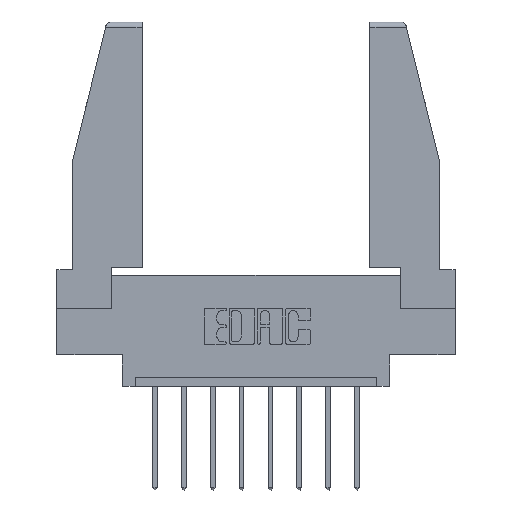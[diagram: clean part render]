
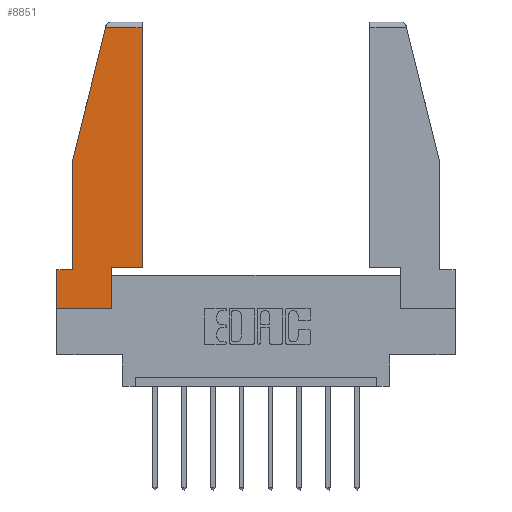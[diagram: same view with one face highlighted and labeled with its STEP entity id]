
A CAD part, top view. The second image highlights one B-rep face of the part: STEP entity #8851.
In plain terms, the highlighted planar face has unit normal (0, 0, 1).
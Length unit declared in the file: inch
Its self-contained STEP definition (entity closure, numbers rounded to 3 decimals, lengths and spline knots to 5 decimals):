
#19 = ORIENTED_EDGE ( 'NONE', *, *, #1486, .T. ) ;
#105 = CARTESIAN_POINT ( 'NONE',  ( 0.297, 0.223, 0. ) ) ;
#138 = LINE ( 'NONE', #12350, #1554 ) ;
#540 = ORIENTED_EDGE ( 'NONE', *, *, #1920, .T. ) ;
#546 = DIRECTION ( 'NONE',  ( 1., 0., 0. ) ) ;
#933 = LINE ( 'NONE', #105, #10803 ) ;
#965 = VERTEX_POINT ( 'NONE', #9725 ) ;
#1338 = CARTESIAN_POINT ( 'NONE',  ( 0.461, 0.223, 0. ) ) ;
#1431 = DIRECTION ( 'NONE',  ( 1., 0., 0. ) ) ;
#1440 = CARTESIAN_POINT ( 'NONE',  ( 0., 0.21, 0. ) ) ;
#1448 = ORIENTED_EDGE ( 'NONE', *, *, #9205, .T. ) ;
#1486 = EDGE_CURVE ( 'NONE', #11310, #4873, #933, .T. ) ;
#1554 = VECTOR ( 'NONE', #1431, 39.37008 ) ;
#1853 = VERTEX_POINT ( 'NONE', #2772 ) ;
#1867 = VERTEX_POINT ( 'NONE', #6920 ) ;
#1920 = EDGE_CURVE ( 'NONE', #4439, #10776, #9570, .T. ) ;
#1997 = DIRECTION ( 'NONE',  ( 0., -1., 0. ) ) ;
#2227 = CARTESIAN_POINT ( 'NONE',  ( 0.271, 1.55, 0. ) ) ;
#2746 = VECTOR ( 'NONE', #11327, 39.37008 ) ;
#2772 = CARTESIAN_POINT ( 'NONE',  ( 0.086, 0.8, 0. ) ) ;
#2821 = VECTOR ( 'NONE', #5313, 39.37008 ) ;
#2903 = LINE ( 'NONE', #12611, #7747 ) ;
#2934 = ORIENTED_EDGE ( 'NONE', *, *, #5352, .T. ) ;
#2991 = ORIENTED_EDGE ( 'NONE', *, *, #7728, .T. ) ;
#3120 = CARTESIAN_POINT ( 'NONE',  ( 0.297, 0.223, 0. ) ) ;
#3161 = ORIENTED_EDGE ( 'NONE', *, *, #10008, .T. ) ;
#4141 = CARTESIAN_POINT ( 'NONE',  ( 0., 0.21, 0. ) ) ;
#4324 = CARTESIAN_POINT ( 'NONE',  ( 0., 0., 0. ) ) ;
#4439 = VERTEX_POINT ( 'NONE', #1440 ) ;
#4545 = ORIENTED_EDGE ( 'NONE', *, *, #7522, .T. ) ;
#4787 = DIRECTION ( 'NONE',  ( 0., -1., 0. ) ) ;
#4873 = VERTEX_POINT ( 'NONE', #8014 ) ;
#4969 = VECTOR ( 'NONE', #4787, 39.37008 ) ;
#5190 = ORIENTED_EDGE ( 'NONE', *, *, #10227, .T. ) ;
#5197 = EDGE_CURVE ( 'NONE', #5452, #11310, #2903, .T. ) ;
#5313 = DIRECTION ( 'NONE',  ( -1., 0., 0. ) ) ;
#5352 = EDGE_CURVE ( 'NONE', #1867, #1853, #7886, .T. ) ;
#5452 = VERTEX_POINT ( 'NONE', #11458 ) ;
#5742 = VECTOR ( 'NONE', #9338, 39.37008 ) ;
#5798 = DIRECTION ( 'NONE',  ( 1., 0., 0. ) ) ;
#5985 = VECTOR ( 'NONE', #1997, 39.37008 ) ;
#6368 = LINE ( 'NONE', #1338, #7914 ) ;
#6620 = EDGE_LOOP ( 'NONE', ( #1448, #4545, #2934, #3161, #5190, #540, #2991, #12308, #19 ) ) ;
#6920 = CARTESIAN_POINT ( 'NONE',  ( 0.2636, 1.52, 0. ) ) ;
#7485 = AXIS2_PLACEMENT_3D ( 'NONE', #9847, #8853, #5798 ) ;
#7522 = EDGE_CURVE ( 'NONE', #11764, #1867, #9364, .T. ) ;
#7728 = EDGE_CURVE ( 'NONE', #10776, #5452, #138, .T. ) ;
#7747 = VECTOR ( 'NONE', #10647, 39.37008 ) ;
#7886 = LINE ( 'NONE', #2227, #5742 ) ;
#7914 = VECTOR ( 'NONE', #9333, 39.37008 ) ;
#8014 = CARTESIAN_POINT ( 'NONE',  ( 0.461, 0.223, 0. ) ) ;
#8367 = FACE_OUTER_BOUND ( 'NONE', #6620, .T. ) ;
#8784 = CARTESIAN_POINT ( 'NONE',  ( 0.086, 0.8, 0. ) ) ;
#8851 = ADVANCED_FACE ( 'NONE', ( #8367 ), #12829, .T. ) ;
#8853 = DIRECTION ( 'NONE',  ( 0., 0., 1. ) ) ;
#9107 = CARTESIAN_POINT ( 'NONE',  ( 0., 1.52, 0. ) ) ;
#9205 = EDGE_CURVE ( 'NONE', #4873, #11764, #6368, .T. ) ;
#9333 = DIRECTION ( 'NONE',  ( 0., 1., 0. ) ) ;
#9338 = DIRECTION ( 'NONE',  ( -0.239, -0.971, 0. ) ) ;
#9364 = LINE ( 'NONE', #9107, #2821 ) ;
#9570 = LINE ( 'NONE', #4141, #5985 ) ;
#9725 = CARTESIAN_POINT ( 'NONE',  ( 0.086, 0.21, 0. ) ) ;
#9779 = LINE ( 'NONE', #11285, #2746 ) ;
#9847 = CARTESIAN_POINT ( 'NONE',  ( 0., 0., 0. ) ) ;
#9931 = LINE ( 'NONE', #8784, #4969 ) ;
#10008 = EDGE_CURVE ( 'NONE', #1853, #965, #9931, .T. ) ;
#10227 = EDGE_CURVE ( 'NONE', #965, #4439, #9779, .T. ) ;
#10647 = DIRECTION ( 'NONE',  ( 0., 1., 0. ) ) ;
#10776 = VERTEX_POINT ( 'NONE', #4324 ) ;
#10803 = VECTOR ( 'NONE', #546, 39.37008 ) ;
#11285 = CARTESIAN_POINT ( 'NONE',  ( 0., 0.21, 0. ) ) ;
#11306 = CARTESIAN_POINT ( 'NONE',  ( 0.461, 1.52, 0. ) ) ;
#11310 = VERTEX_POINT ( 'NONE', #3120 ) ;
#11327 = DIRECTION ( 'NONE',  ( -1., 0., 0. ) ) ;
#11458 = CARTESIAN_POINT ( 'NONE',  ( 0.297, 0., 0. ) ) ;
#11764 = VERTEX_POINT ( 'NONE', #11306 ) ;
#12308 = ORIENTED_EDGE ( 'NONE', *, *, #5197, .T. ) ;
#12350 = CARTESIAN_POINT ( 'NONE',  ( 0., 0., 0. ) ) ;
#12611 = CARTESIAN_POINT ( 'NONE',  ( 0.297, 0., 0. ) ) ;
#12829 = PLANE ( 'NONE',  #7485 ) ;
